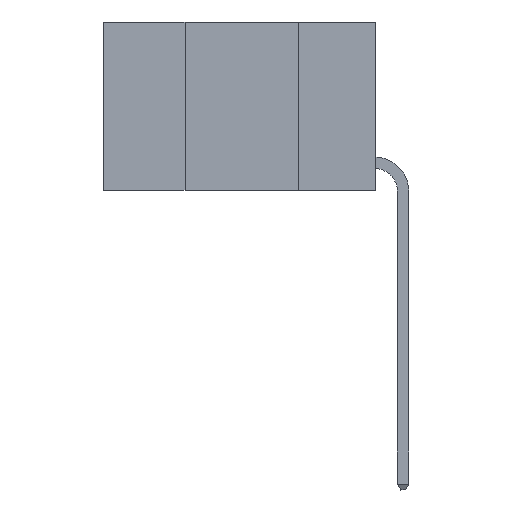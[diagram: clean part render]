
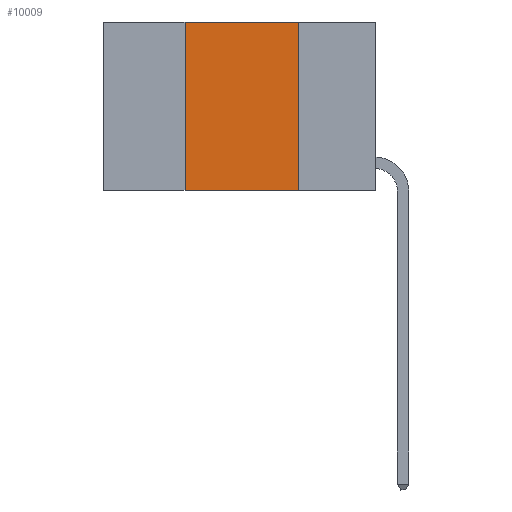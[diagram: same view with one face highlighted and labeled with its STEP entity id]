
A CAD part, left-side view. The second image highlights one B-rep face of the part: STEP entity #10009.
In plain terms, the highlighted planar face has unit normal (-1, 0, 0).
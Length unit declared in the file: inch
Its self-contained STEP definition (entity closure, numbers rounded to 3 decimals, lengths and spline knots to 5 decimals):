
#73 = CARTESIAN_POINT ( 'NONE',  ( 0., 0.42, 0. ) ) ;
#183 = ORIENTED_EDGE ( 'NONE', *, *, #12778, .F. ) ;
#333 = EDGE_CURVE ( 'NONE', #7975, #5344, #4998, .T. ) ;
#1677 = CARTESIAN_POINT ( 'NONE',  ( 0., 0.6, 0. ) ) ;
#2485 = VECTOR ( 'NONE', #21756, 39.37008 ) ;
#3673 = EDGE_CURVE ( 'NONE', #7975, #15434, #13442, .T. ) ;
#3737 = CARTESIAN_POINT ( 'NONE',  ( 0., 0.17, -0.37 ) ) ;
#3994 = CARTESIAN_POINT ( 'NONE',  ( 0., 0.6, -0.37 ) ) ;
#4329 = FACE_OUTER_BOUND ( 'NONE', #17693, .T. ) ;
#4998 = LINE ( 'NONE', #19952, #5894 ) ;
#5344 = VERTEX_POINT ( 'NONE', #73 ) ;
#5894 = VECTOR ( 'NONE', #14565, 39.37008 ) ;
#6417 = EDGE_CURVE ( 'NONE', #12514, #15434, #12420, .T. ) ;
#6727 = DIRECTION ( 'NONE',  ( 1., 0., 0. ) ) ;
#6991 = PLANE ( 'NONE',  #20936 ) ;
#7975 = VERTEX_POINT ( 'NONE', #15216 ) ;
#10004 = ORIENTED_EDGE ( 'NONE', *, *, #333, .F. ) ;
#10009 = ADVANCED_FACE ( 'NONE', ( #4329 ), #6991, .F. ) ;
#11983 = VECTOR ( 'NONE', #21053, 39.37008 ) ;
#12242 = CARTESIAN_POINT ( 'NONE',  ( 0., 0.17, 0. ) ) ;
#12420 = LINE ( 'NONE', #17940, #2485 ) ;
#12514 = VERTEX_POINT ( 'NONE', #12242 ) ;
#12778 = EDGE_CURVE ( 'NONE', #5344, #12514, #15137, .T. ) ;
#13442 = LINE ( 'NONE', #3994, #18115 ) ;
#14565 = DIRECTION ( 'NONE',  ( 0., 0., 1. ) ) ;
#15137 = LINE ( 'NONE', #1677, #11983 ) ;
#15216 = CARTESIAN_POINT ( 'NONE',  ( 0., 0.42, -0.37 ) ) ;
#15434 = VERTEX_POINT ( 'NONE', #3737 ) ;
#16495 = DIRECTION ( 'NONE',  ( 0., 0., -1. ) ) ;
#17356 = ORIENTED_EDGE ( 'NONE', *, *, #6417, .F. ) ;
#17693 = EDGE_LOOP ( 'NONE', ( #17356, #183, #10004, #22324 ) ) ;
#17940 = CARTESIAN_POINT ( 'NONE',  ( 0., 0.17, 0. ) ) ;
#18115 = VECTOR ( 'NONE', #19206, 39.37008 ) ;
#18499 = CARTESIAN_POINT ( 'NONE',  ( 0., 0.6, 0. ) ) ;
#19206 = DIRECTION ( 'NONE',  ( 0., -1., 0. ) ) ;
#19952 = CARTESIAN_POINT ( 'NONE',  ( 0., 0.42, 0. ) ) ;
#20936 = AXIS2_PLACEMENT_3D ( 'NONE', #18499, #6727, #16495 ) ;
#21053 = DIRECTION ( 'NONE',  ( 0., -1., 0. ) ) ;
#21756 = DIRECTION ( 'NONE',  ( 0., 0., -1. ) ) ;
#22324 = ORIENTED_EDGE ( 'NONE', *, *, #3673, .T. ) ;
